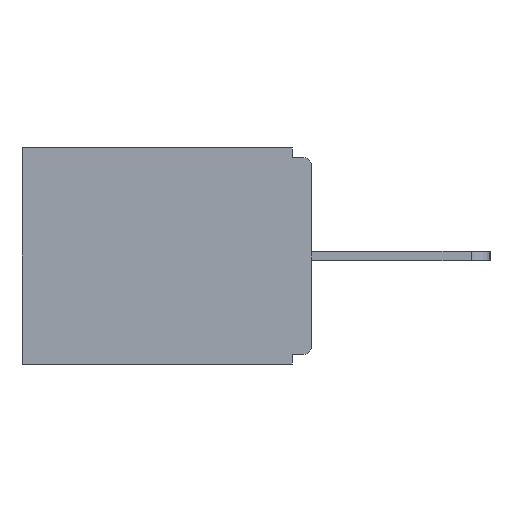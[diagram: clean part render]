
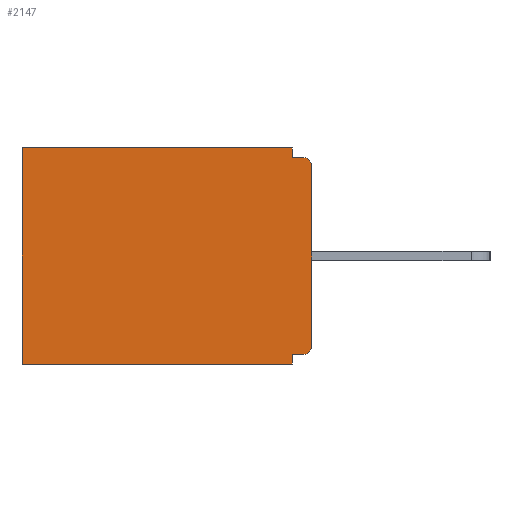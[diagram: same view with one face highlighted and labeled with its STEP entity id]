
A CAD part, left-side view. The second image highlights one B-rep face of the part: STEP entity #2147.
In plain terms, the highlighted planar face has unit normal (-1, 0, 0).
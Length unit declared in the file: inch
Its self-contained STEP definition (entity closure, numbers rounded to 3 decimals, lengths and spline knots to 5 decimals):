
#428 = VERTEX_POINT ( 'NONE', #9716 ) ;
#565 = LINE ( 'NONE', #18228, #4498 ) ;
#691 = DIRECTION ( 'NONE',  ( 0., 0., -1. ) ) ;
#758 = DIRECTION ( 'NONE',  ( 0., 0., -1. ) ) ;
#878 = ORIENTED_EDGE ( 'NONE', *, *, #9526, .F. ) ;
#892 = ORIENTED_EDGE ( 'NONE', *, *, #7437, .T. ) ;
#923 = LINE ( 'NONE', #12907, #9109 ) ;
#1437 = ORIENTED_EDGE ( 'NONE', *, *, #3198, .T. ) ;
#2087 = EDGE_CURVE ( 'NONE', #7921, #20276, #923, .T. ) ;
#2147 = ADVANCED_FACE ( 'NONE', ( #15986 ), #11880, .F. ) ;
#2150 = VERTEX_POINT ( 'NONE', #14849 ) ;
#2729 = CIRCLE ( 'NONE', #19718, 0.015 ) ;
#2887 = CARTESIAN_POINT ( 'NONE',  ( 0.298, 0., -0.015 ) ) ;
#3198 = EDGE_CURVE ( 'NONE', #19376, #428, #2729, .T. ) ;
#3265 = VECTOR ( 'NONE', #8587, 39.37008 ) ;
#3297 = LINE ( 'NONE', #7427, #8150 ) ;
#3821 = VECTOR ( 'NONE', #14037, 39.37008 ) ;
#3855 = VERTEX_POINT ( 'NONE', #10719 ) ;
#4205 = ORIENTED_EDGE ( 'NONE', *, *, #19605, .T. ) ;
#4231 = LINE ( 'NONE', #4939, #8525 ) ;
#4309 = LINE ( 'NONE', #16378, #3265 ) ;
#4498 = VECTOR ( 'NONE', #691, 39.37008 ) ;
#4939 = CARTESIAN_POINT ( 'NONE',  ( 0.298, 0., -0.343 ) ) ;
#5276 = ORIENTED_EDGE ( 'NONE', *, *, #19943, .F. ) ;
#5499 = VERTEX_POINT ( 'NONE', #5792 ) ;
#5532 = DIRECTION ( 'NONE',  ( 0., 0., -1. ) ) ;
#5792 = CARTESIAN_POINT ( 'NONE',  ( 0.298, 0.015, -0.328 ) ) ;
#5910 = EDGE_CURVE ( 'NONE', #2150, #20384, #14343, .T. ) ;
#7146 = ORIENTED_EDGE ( 'NONE', *, *, #19772, .F. ) ;
#7427 = CARTESIAN_POINT ( 'NONE',  ( 0.298, 0.031, -0.343 ) ) ;
#7437 = EDGE_CURVE ( 'NONE', #5499, #11629, #15296, .T. ) ;
#7478 = ORIENTED_EDGE ( 'NONE', *, *, #2087, .T. ) ;
#7793 = DIRECTION ( 'NONE',  ( 0., 1., 0. ) ) ;
#7802 = ORIENTED_EDGE ( 'NONE', *, *, #5910, .F. ) ;
#7921 = VERTEX_POINT ( 'NONE', #15819 ) ;
#8150 = VECTOR ( 'NONE', #758, 39.37008 ) ;
#8525 = VECTOR ( 'NONE', #15978, 39.37008 ) ;
#8587 = DIRECTION ( 'NONE',  ( 0., 1., 0. ) ) ;
#8821 = DIRECTION ( 'NONE',  ( 1., 0., 0. ) ) ;
#9109 = VECTOR ( 'NONE', #15079, 39.37008 ) ;
#9112 = ORIENTED_EDGE ( 'NONE', *, *, #11195, .F. ) ;
#9404 = AXIS2_PLACEMENT_3D ( 'NONE', #20236, #8821, #13591 ) ;
#9526 = EDGE_CURVE ( 'NONE', #20384, #428, #16447, .T. ) ;
#9716 = CARTESIAN_POINT ( 'NONE',  ( 0.298, 0.015, -0.015 ) ) ;
#10169 = VECTOR ( 'NONE', #5532, 39.37008 ) ;
#10719 = CARTESIAN_POINT ( 'NONE',  ( 0.298, 0.031, -0.343 ) ) ;
#10899 = EDGE_LOOP ( 'NONE', ( #1437, #878, #7802, #4205, #7478, #7146, #18126, #5276, #892, #9112 ) ) ;
#11195 = EDGE_CURVE ( 'NONE', #19376, #11629, #565, .T. ) ;
#11200 = CARTESIAN_POINT ( 'NONE',  ( 0.298, 0.031, -0.343 ) ) ;
#11418 = VECTOR ( 'NONE', #7793, 39.37008 ) ;
#11629 = VERTEX_POINT ( 'NONE', #16832 ) ;
#11653 = CARTESIAN_POINT ( 'NONE',  ( 0.298, 0.015, -0.313 ) ) ;
#11705 = CARTESIAN_POINT ( 'NONE',  ( 0.298, 0., -0.03 ) ) ;
#11880 = PLANE ( 'NONE',  #9404 ) ;
#12405 = CARTESIAN_POINT ( 'NONE',  ( 0.298, 0., 0. ) ) ;
#12440 = DIRECTION ( 'NONE',  ( -1., 0., 0. ) ) ;
#12446 = DIRECTION ( 'NONE',  ( 0., 0., -1. ) ) ;
#12709 = CARTESIAN_POINT ( 'NONE',  ( 0.298, 0.015, -0.03 ) ) ;
#12713 = DIRECTION ( 'NONE',  ( -1., 0., 0. ) ) ;
#12727 = DIRECTION ( 'NONE',  ( 0., 0., -1. ) ) ;
#12907 = CARTESIAN_POINT ( 'NONE',  ( 0.298, 0.46, 0. ) ) ;
#13591 = DIRECTION ( 'NONE',  ( 0., 0., -1. ) ) ;
#14037 = DIRECTION ( 'NONE',  ( 0., -1., 0. ) ) ;
#14216 = VERTEX_POINT ( 'NONE', #18758 ) ;
#14343 = LINE ( 'NONE', #11200, #10169 ) ;
#14849 = CARTESIAN_POINT ( 'NONE',  ( 0.298, 0.031, 0. ) ) ;
#15079 = DIRECTION ( 'NONE',  ( 0., 0., -1. ) ) ;
#15296 = CIRCLE ( 'NONE', #17692, 0.015 ) ;
#15618 = LINE ( 'NONE', #12405, #11418 ) ;
#15819 = CARTESIAN_POINT ( 'NONE',  ( 0.298, 0.46, 0. ) ) ;
#15978 = DIRECTION ( 'NONE',  ( 0., 1., 0. ) ) ;
#15986 = FACE_OUTER_BOUND ( 'NONE', #10899, .T. ) ;
#16378 = CARTESIAN_POINT ( 'NONE',  ( 0.298, 0., -0.328 ) ) ;
#16447 = LINE ( 'NONE', #2887, #3821 ) ;
#16832 = CARTESIAN_POINT ( 'NONE',  ( 0.298, 0., -0.313 ) ) ;
#17692 = AXIS2_PLACEMENT_3D ( 'NONE', #11653, #12440, #12446 ) ;
#17704 = CARTESIAN_POINT ( 'NONE',  ( 0.298, 0.46, -0.343 ) ) ;
#17785 = EDGE_CURVE ( 'NONE', #14216, #3855, #3297, .T. ) ;
#17972 = CARTESIAN_POINT ( 'NONE',  ( 0.298, 0.031, -0.015 ) ) ;
#18126 = ORIENTED_EDGE ( 'NONE', *, *, #17785, .F. ) ;
#18228 = CARTESIAN_POINT ( 'NONE',  ( 0.298, 0., 0. ) ) ;
#18758 = CARTESIAN_POINT ( 'NONE',  ( 0.298, 0.031, -0.328 ) ) ;
#19376 = VERTEX_POINT ( 'NONE', #11705 ) ;
#19605 = EDGE_CURVE ( 'NONE', #2150, #7921, #15618, .T. ) ;
#19718 = AXIS2_PLACEMENT_3D ( 'NONE', #12709, #12713, #12727 ) ;
#19772 = EDGE_CURVE ( 'NONE', #3855, #20276, #4231, .T. ) ;
#19943 = EDGE_CURVE ( 'NONE', #5499, #14216, #4309, .T. ) ;
#20236 = CARTESIAN_POINT ( 'NONE',  ( 0.298, 0., 0. ) ) ;
#20276 = VERTEX_POINT ( 'NONE', #17704 ) ;
#20384 = VERTEX_POINT ( 'NONE', #17972 ) ;
